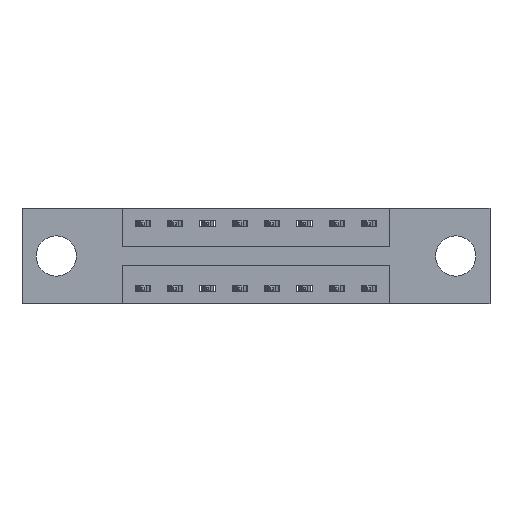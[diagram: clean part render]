
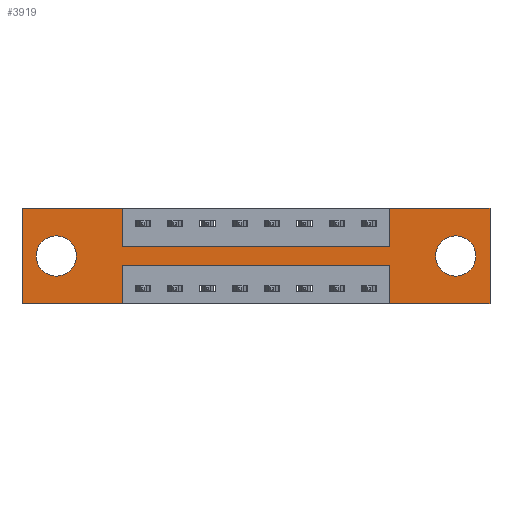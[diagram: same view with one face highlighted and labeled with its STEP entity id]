
A CAD part, front view. The second image highlights one B-rep face of the part: STEP entity #3919.
In plain terms, the highlighted planar face has unit normal (0, -1, 0).
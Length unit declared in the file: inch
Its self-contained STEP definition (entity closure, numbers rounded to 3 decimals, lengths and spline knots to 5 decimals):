
#17 = CARTESIAN_POINT ( 'NONE',  ( 1.4225, 0., -0.15 ) ) ;
#24 = VERTEX_POINT ( 'NONE', #9735 ) ;
#60 = DIRECTION ( 'NONE',  ( -1., 0., 0. ) ) ;
#207 = VERTEX_POINT ( 'NONE', #2002 ) ;
#273 = FACE_OUTER_BOUND ( 'NONE', #9360, .T. ) ;
#286 = ORIENTED_EDGE ( 'NONE', *, *, #6168, .F. ) ;
#382 = AXIS2_PLACEMENT_3D ( 'NONE', #7462, #2708, #5870 ) ;
#388 = LINE ( 'NONE', #4497, #4167 ) ;
#440 = DIRECTION ( 'NONE',  ( 0., 0., -1. ) ) ;
#492 = CARTESIAN_POINT ( 'NONE',  ( 0.3875, 0., -0.15 ) ) ;
#570 = CARTESIAN_POINT ( 'NONE',  ( 1.4225, 0., -0.22 ) ) ;
#589 = CARTESIAN_POINT ( 'NONE',  ( 0.3875, 0., -0.15 ) ) ;
#639 = ORIENTED_EDGE ( 'NONE', *, *, #3589, .F. ) ;
#653 = CARTESIAN_POINT ( 'NONE',  ( 1.6775, 0., -0.185 ) ) ;
#876 = ORIENTED_EDGE ( 'NONE', *, *, #7470, .F. ) ;
#922 = VECTOR ( 'NONE', #2224, 39.37008 ) ;
#949 = DIRECTION ( 'NONE',  ( 0., 1., 0. ) ) ;
#988 = CARTESIAN_POINT ( 'NONE',  ( 0., 0., -0.37 ) ) ;
#993 = VECTOR ( 'NONE', #9303, 39.37008 ) ;
#1053 = DIRECTION ( 'NONE',  ( 0., 0., -1. ) ) ;
#1153 = DIRECTION ( 'NONE',  ( 0., 0., -1. ) ) ;
#1355 = EDGE_CURVE ( 'NONE', #4904, #4117, #5321, .T. ) ;
#1422 = ORIENTED_EDGE ( 'NONE', *, *, #2469, .F. ) ;
#1680 = AXIS2_PLACEMENT_3D ( 'NONE', #1948, #8246, #1153 ) ;
#1682 = LINE ( 'NONE', #8915, #2851 ) ;
#1800 = CARTESIAN_POINT ( 'NONE',  ( 0.3875, 0., -0.22 ) ) ;
#1831 = EDGE_LOOP ( 'NONE', ( #2188, #6490 ) ) ;
#1895 = CARTESIAN_POINT ( 'NONE',  ( 1.81, 0., 0. ) ) ;
#1908 = CIRCLE ( 'NONE', #382, 0.078 ) ;
#1928 = VERTEX_POINT ( 'NONE', #1800 ) ;
#1948 = CARTESIAN_POINT ( 'NONE',  ( 0., 0., -0.37 ) ) ;
#2002 = CARTESIAN_POINT ( 'NONE',  ( 1.6775, 0., -0.263 ) ) ;
#2017 = CARTESIAN_POINT ( 'NONE',  ( 1.4225, 0., -0.37 ) ) ;
#2040 = ORIENTED_EDGE ( 'NONE', *, *, #9235, .F. ) ;
#2153 = AXIS2_PLACEMENT_3D ( 'NONE', #3237, #949, #2553 ) ;
#2188 = ORIENTED_EDGE ( 'NONE', *, *, #4945, .T. ) ;
#2224 = DIRECTION ( 'NONE',  ( 0., 0., 1. ) ) ;
#2274 = LINE ( 'NONE', #6863, #922 ) ;
#2469 = EDGE_CURVE ( 'NONE', #4117, #10076, #5781, .T. ) ;
#2495 = CIRCLE ( 'NONE', #9461, 0.078 ) ;
#2553 = DIRECTION ( 'NONE',  ( 0., 0., 1. ) ) ;
#2708 = DIRECTION ( 'NONE',  ( 0., 1., 0. ) ) ;
#2767 = CARTESIAN_POINT ( 'NONE',  ( 0., 0., -0.37 ) ) ;
#2851 = VECTOR ( 'NONE', #9565, 39.37008 ) ;
#2861 = VECTOR ( 'NONE', #8283, 39.37008 ) ;
#2895 = CARTESIAN_POINT ( 'NONE',  ( 0., 0., -0.37 ) ) ;
#2994 = ORIENTED_EDGE ( 'NONE', *, *, #3878, .F. ) ;
#3167 = ORIENTED_EDGE ( 'NONE', *, *, #4246, .F. ) ;
#3237 = CARTESIAN_POINT ( 'NONE',  ( 0.1325, 0., -0.185 ) ) ;
#3258 = VECTOR ( 'NONE', #9872, 39.37008 ) ;
#3461 = ORIENTED_EDGE ( 'NONE', *, *, #9337, .F. ) ;
#3552 = VERTEX_POINT ( 'NONE', #6814 ) ;
#3584 = VERTEX_POINT ( 'NONE', #8752 ) ;
#3589 = EDGE_CURVE ( 'NONE', #24, #7710, #9260, .T. ) ;
#3611 = LINE ( 'NONE', #2895, #3891 ) ;
#3681 = VECTOR ( 'NONE', #8721, 39.37008 ) ;
#3714 = DIRECTION ( 'NONE',  ( 1., 0., 0. ) ) ;
#3762 = ORIENTED_EDGE ( 'NONE', *, *, #4217, .T. ) ;
#3776 = CARTESIAN_POINT ( 'NONE',  ( 0., 0., 0. ) ) ;
#3804 = VECTOR ( 'NONE', #1053, 39.37008 ) ;
#3878 = EDGE_CURVE ( 'NONE', #5667, #4440, #6634, .T. ) ;
#3891 = VECTOR ( 'NONE', #9898, 39.37008 ) ;
#3919 = ADVANCED_FACE ( 'NONE', ( #7373, #5832, #273 ), #5876, .T. ) ;
#4117 = VERTEX_POINT ( 'NONE', #17 ) ;
#4167 = VECTOR ( 'NONE', #3714, 39.37008 ) ;
#4171 = CARTESIAN_POINT ( 'NONE',  ( 1.4225, 0., 0. ) ) ;
#4217 = EDGE_CURVE ( 'NONE', #10158, #9446, #6448, .T. ) ;
#4246 = EDGE_CURVE ( 'NONE', #3584, #4904, #5141, .T. ) ;
#4414 = DIRECTION ( 'NONE',  ( 0., 0., -1. ) ) ;
#4440 = VERTEX_POINT ( 'NONE', #9130 ) ;
#4497 = CARTESIAN_POINT ( 'NONE',  ( 0., 0., 0. ) ) ;
#4499 = CARTESIAN_POINT ( 'NONE',  ( 0.1325, 0., -0.107 ) ) ;
#4640 = AXIS2_PLACEMENT_3D ( 'NONE', #8368, #9112, #440 ) ;
#4843 = CARTESIAN_POINT ( 'NONE',  ( 1.81, 0., 0. ) ) ;
#4904 = VERTEX_POINT ( 'NONE', #492 ) ;
#4932 = CARTESIAN_POINT ( 'NONE',  ( 0.3875, 0., 0. ) ) ;
#4945 = EDGE_CURVE ( 'NONE', #8078, #207, #9781, .T. ) ;
#5141 = LINE ( 'NONE', #4932, #3804 ) ;
#5175 = DIRECTION ( 'NONE',  ( 0., 0., 1. ) ) ;
#5321 = LINE ( 'NONE', #589, #993 ) ;
#5487 = EDGE_CURVE ( 'NONE', #207, #8078, #2495, .T. ) ;
#5667 = VERTEX_POINT ( 'NONE', #4843 ) ;
#5745 = EDGE_LOOP ( 'NONE', ( #3762, #9797 ) ) ;
#5781 = LINE ( 'NONE', #4171, #3258 ) ;
#5832 = FACE_BOUND ( 'NONE', #5745, .T. ) ;
#5870 = DIRECTION ( 'NONE',  ( 0., 0., 1. ) ) ;
#5872 = VECTOR ( 'NONE', #60, 39.37008 ) ;
#5876 = PLANE ( 'NONE',  #1680 ) ;
#5917 = LINE ( 'NONE', #6778, #2861 ) ;
#6062 = VERTEX_POINT ( 'NONE', #3776 ) ;
#6142 = VECTOR ( 'NONE', #4414, 39.37008 ) ;
#6168 = EDGE_CURVE ( 'NONE', #10076, #5667, #388, .T. ) ;
#6233 = LINE ( 'NONE', #8617, #3681 ) ;
#6309 = VECTOR ( 'NONE', #5175, 39.37008 ) ;
#6360 = DIRECTION ( 'NONE',  ( 0., 0., -1. ) ) ;
#6448 = CIRCLE ( 'NONE', #2153, 0.078 ) ;
#6490 = ORIENTED_EDGE ( 'NONE', *, *, #5487, .T. ) ;
#6634 = LINE ( 'NONE', #1895, #6142 ) ;
#6778 = CARTESIAN_POINT ( 'NONE',  ( 0.3875, 0., -0.37 ) ) ;
#6814 = CARTESIAN_POINT ( 'NONE',  ( 0.3875, 0., -0.37 ) ) ;
#6863 = CARTESIAN_POINT ( 'NONE',  ( 0., 0., 0. ) ) ;
#7101 = ORIENTED_EDGE ( 'NONE', *, *, #9919, .F. ) ;
#7275 = EDGE_CURVE ( 'NONE', #7710, #1928, #1682, .T. ) ;
#7373 = FACE_BOUND ( 'NONE', #1831, .T. ) ;
#7462 = CARTESIAN_POINT ( 'NONE',  ( 0.1325, 0., -0.185 ) ) ;
#7470 = EDGE_CURVE ( 'NONE', #1928, #3552, #5917, .T. ) ;
#7501 = CARTESIAN_POINT ( 'NONE',  ( 1.4225, 0., 0. ) ) ;
#7710 = VERTEX_POINT ( 'NONE', #570 ) ;
#7750 = EDGE_CURVE ( 'NONE', #6062, #3584, #6233, .T. ) ;
#7861 = DIRECTION ( 'NONE',  ( 0., 1., 0. ) ) ;
#8078 = VERTEX_POINT ( 'NONE', #9897 ) ;
#8246 = DIRECTION ( 'NONE',  ( 0., -1., 0. ) ) ;
#8283 = DIRECTION ( 'NONE',  ( 0., 0., -1. ) ) ;
#8368 = CARTESIAN_POINT ( 'NONE',  ( 1.6775, 0., -0.185 ) ) ;
#8459 = VERTEX_POINT ( 'NONE', #2767 ) ;
#8617 = CARTESIAN_POINT ( 'NONE',  ( 0., 0., 0. ) ) ;
#8717 = ORIENTED_EDGE ( 'NONE', *, *, #1355, .F. ) ;
#8721 = DIRECTION ( 'NONE',  ( 1., 0., 0. ) ) ;
#8752 = CARTESIAN_POINT ( 'NONE',  ( 0.3875, 0., 0. ) ) ;
#8915 = CARTESIAN_POINT ( 'NONE',  ( 0.3875, 0., -0.22 ) ) ;
#8992 = EDGE_CURVE ( 'NONE', #9446, #10158, #1908, .T. ) ;
#9112 = DIRECTION ( 'NONE',  ( 0., 1., 0. ) ) ;
#9130 = CARTESIAN_POINT ( 'NONE',  ( 1.81, 0., -0.37 ) ) ;
#9235 = EDGE_CURVE ( 'NONE', #4440, #24, #9595, .T. ) ;
#9260 = LINE ( 'NONE', #2017, #6309 ) ;
#9303 = DIRECTION ( 'NONE',  ( 1., 0., 0. ) ) ;
#9337 = EDGE_CURVE ( 'NONE', #3552, #8459, #3611, .T. ) ;
#9360 = EDGE_LOOP ( 'NONE', ( #876, #10064, #639, #2040, #2994, #286, #1422, #8717, #3167, #9746, #7101, #3461 ) ) ;
#9435 = CARTESIAN_POINT ( 'NONE',  ( 0.1325, 0., -0.263 ) ) ;
#9446 = VERTEX_POINT ( 'NONE', #9435 ) ;
#9461 = AXIS2_PLACEMENT_3D ( 'NONE', #653, #7861, #6360 ) ;
#9565 = DIRECTION ( 'NONE',  ( -1., 0., 0. ) ) ;
#9595 = LINE ( 'NONE', #988, #5872 ) ;
#9735 = CARTESIAN_POINT ( 'NONE',  ( 1.4225, 0., -0.37 ) ) ;
#9746 = ORIENTED_EDGE ( 'NONE', *, *, #7750, .F. ) ;
#9781 = CIRCLE ( 'NONE', #4640, 0.078 ) ;
#9797 = ORIENTED_EDGE ( 'NONE', *, *, #8992, .T. ) ;
#9872 = DIRECTION ( 'NONE',  ( 0., 0., 1. ) ) ;
#9897 = CARTESIAN_POINT ( 'NONE',  ( 1.6775, 0., -0.107 ) ) ;
#9898 = DIRECTION ( 'NONE',  ( -1., 0., 0. ) ) ;
#9919 = EDGE_CURVE ( 'NONE', #8459, #6062, #2274, .T. ) ;
#10064 = ORIENTED_EDGE ( 'NONE', *, *, #7275, .F. ) ;
#10076 = VERTEX_POINT ( 'NONE', #7501 ) ;
#10158 = VERTEX_POINT ( 'NONE', #4499 ) ;
